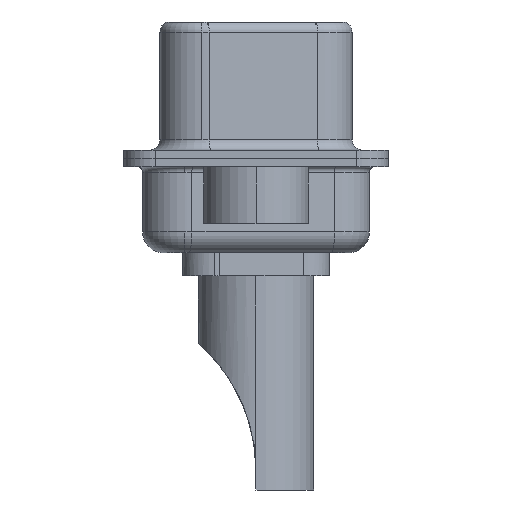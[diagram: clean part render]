
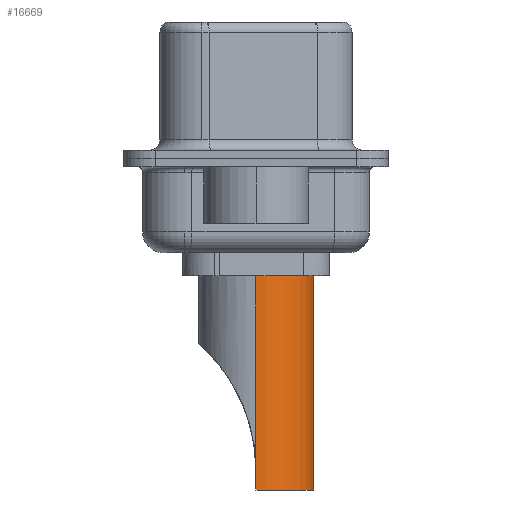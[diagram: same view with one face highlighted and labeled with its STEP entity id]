
A CAD part, left-side view. The second image highlights one B-rep face of the part: STEP entity #16669.
In plain terms, the highlighted cylindrical face has radius 2.75 mm (diameter 5.5 mm), a partial arc.
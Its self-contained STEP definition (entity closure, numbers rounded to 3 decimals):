
#109 = CARTESIAN_POINT ( 'NONE',  ( 2.75, 0., 4.234 ) ) ;
#669 = DIRECTION ( 'NONE',  ( 0., 0., 1. ) ) ;
#720 = AXIS2_PLACEMENT_3D ( 'NONE', #763, #12693, #14176 ) ;
#763 = CARTESIAN_POINT ( 'NONE',  ( 0., 0., 1.5 ) ) ;
#1520 = CARTESIAN_POINT ( 'NONE',  ( -2.75, 0., -8.7 ) ) ;
#2534 = CARTESIAN_POINT ( 'NONE',  ( 0., 0., 4.234 ) ) ;
#3091 = CARTESIAN_POINT ( 'NONE',  ( 2.75, 0., -8.7 ) ) ;
#3307 = EDGE_CURVE ( 'NONE', #10463, #15337, #4394, .T. ) ;
#3770 = CYLINDRICAL_SURFACE ( 'NONE', #8291, 2.75 ) ;
#3965 = EDGE_CURVE ( 'NONE', #10463, #18367, #8710, .T. ) ;
#3998 = VERTEX_POINT ( 'NONE', #14622 ) ;
#4394 = LINE ( 'NONE', #3091, #12351 ) ;
#4652 = FACE_OUTER_BOUND ( 'NONE', #14423, .T. ) ;
#4665 = DIRECTION ( 'NONE',  ( 0., 0., 1. ) ) ;
#6057 = CARTESIAN_POINT ( 'NONE',  ( 2.75, 0., 1.5 ) ) ;
#6060 = CIRCLE ( 'NONE', #720, 2.75 ) ;
#6267 = VECTOR ( 'NONE', #669, 1000. ) ;
#6397 = ORIENTED_EDGE ( 'NONE', *, *, #11036, .T. ) ;
#6718 = LINE ( 'NONE', #1520, #10090 ) ;
#6972 = AXIS2_PLACEMENT_3D ( 'NONE', #12928, #14211, #14343 ) ;
#7567 = VECTOR ( 'NONE', #4665, 1000. ) ;
#8291 = AXIS2_PLACEMENT_3D ( 'NONE', #2534, #11280, #8426 ) ;
#8426 = DIRECTION ( 'NONE',  ( 1., 0., 0. ) ) ;
#8690 = EDGE_CURVE ( 'NONE', #11892, #18367, #6060, .T. ) ;
#8710 = LINE ( 'NONE', #109, #7567 ) ;
#9092 = CARTESIAN_POINT ( 'NONE',  ( 2.75, 0., -8.7 ) ) ;
#10090 = VECTOR ( 'NONE', #14721, 1000. ) ;
#10189 = CARTESIAN_POINT ( 'NONE',  ( -2.75, 0., -8.7 ) ) ;
#10463 = VERTEX_POINT ( 'NONE', #17648 ) ;
#10669 = ORIENTED_EDGE ( 'NONE', *, *, #3307, .F. ) ;
#10906 = CARTESIAN_POINT ( 'NONE',  ( -2.75, 0., 4.234 ) ) ;
#11036 = EDGE_CURVE ( 'NONE', #14987, #15337, #12088, .T. ) ;
#11280 = DIRECTION ( 'NONE',  ( 0., 0., 1. ) ) ;
#11892 = VERTEX_POINT ( 'NONE', #17927 ) ;
#11924 = DIRECTION ( 'NONE',  ( 0., 0., -1. ) ) ;
#12088 = CIRCLE ( 'NONE', #6972, 2.75 ) ;
#12186 = ORIENTED_EDGE ( 'NONE', *, *, #3965, .T. ) ;
#12351 = VECTOR ( 'NONE', #11924, 1000. ) ;
#12693 = DIRECTION ( 'NONE',  ( 0., 0., 1. ) ) ;
#12928 = CARTESIAN_POINT ( 'NONE',  ( 0., 0., -8.7 ) ) ;
#14176 = DIRECTION ( 'NONE',  ( 1., 0., 0. ) ) ;
#14211 = DIRECTION ( 'NONE',  ( 0., 0., 1. ) ) ;
#14343 = DIRECTION ( 'NONE',  ( 1., 0., 0. ) ) ;
#14423 = EDGE_LOOP ( 'NONE', ( #17923, #15503, #6397, #10669, #12186, #15896 ) ) ;
#14622 = CARTESIAN_POINT ( 'NONE',  ( -2.75, 0., -7.764 ) ) ;
#14721 = DIRECTION ( 'NONE',  ( 0., 0., -1. ) ) ;
#14987 = VERTEX_POINT ( 'NONE', #10189 ) ;
#15337 = VERTEX_POINT ( 'NONE', #9092 ) ;
#15503 = ORIENTED_EDGE ( 'NONE', *, *, #16816, .T. ) ;
#15896 = ORIENTED_EDGE ( 'NONE', *, *, #8690, .F. ) ;
#16101 = EDGE_CURVE ( 'NONE', #3998, #11892, #17186, .T. ) ;
#16669 = ADVANCED_FACE ( 'NONE', ( #4652 ), #3770, .T. ) ;
#16816 = EDGE_CURVE ( 'NONE', #3998, #14987, #6718, .T. ) ;
#17186 = LINE ( 'NONE', #10906, #6267 ) ;
#17648 = CARTESIAN_POINT ( 'NONE',  ( 2.75, 0., -7.764 ) ) ;
#17923 = ORIENTED_EDGE ( 'NONE', *, *, #16101, .F. ) ;
#17927 = CARTESIAN_POINT ( 'NONE',  ( -2.75, 0., 1.5 ) ) ;
#18367 = VERTEX_POINT ( 'NONE', #6057 ) ;
